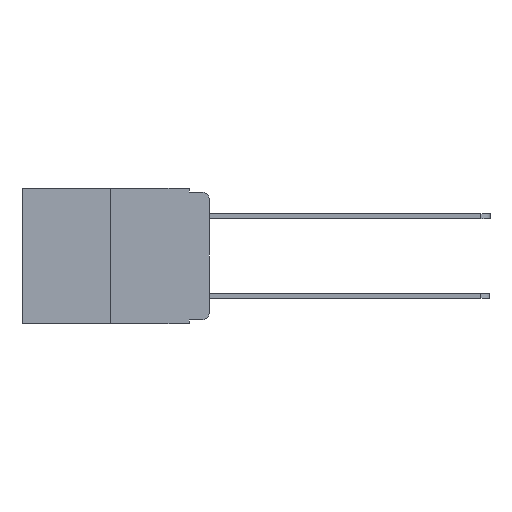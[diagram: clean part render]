
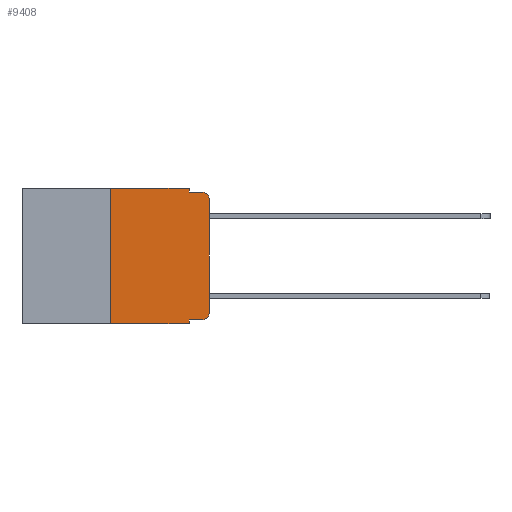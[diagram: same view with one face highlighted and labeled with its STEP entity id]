
A CAD part, left-side view. The second image highlights one B-rep face of the part: STEP entity #9408.
In plain terms, the highlighted planar face has unit normal (-1, 0, 0).
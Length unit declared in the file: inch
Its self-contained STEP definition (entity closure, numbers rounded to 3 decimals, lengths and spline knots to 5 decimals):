
#46 = DIRECTION ( 'NONE',  ( 0., -1., 0. ) ) ;
#135 = EDGE_CURVE ( 'NONE', #862, #12136, #13239, .T. ) ;
#237 = CARTESIAN_POINT ( 'NONE',  ( 0., 0.051, -0.333 ) ) ;
#331 = CIRCLE ( 'NONE', #6655, 0.02 ) ;
#479 = LINE ( 'NONE', #8458, #13839 ) ;
#651 = VERTEX_POINT ( 'NONE', #237 ) ;
#794 = VECTOR ( 'NONE', #2720, 39.37008 ) ;
#862 = VERTEX_POINT ( 'NONE', #13949 ) ;
#1198 = CARTESIAN_POINT ( 'NONE',  ( 0., 0., -0.03 ) ) ;
#1279 = CARTESIAN_POINT ( 'NONE',  ( 0., 0., -0.313 ) ) ;
#1744 = CARTESIAN_POINT ( 'NONE',  ( 0., 0., 0. ) ) ;
#1793 = CARTESIAN_POINT ( 'NONE',  ( 0., 0.051, -0.01 ) ) ;
#2122 = DIRECTION ( 'NONE',  ( 0., 0., -1. ) ) ;
#2189 = DIRECTION ( 'NONE',  ( 0., 0., -1. ) ) ;
#2307 = EDGE_CURVE ( 'NONE', #651, #6508, #14118, .T. ) ;
#2720 = DIRECTION ( 'NONE',  ( 0., 0., -1. ) ) ;
#2886 = EDGE_CURVE ( 'NONE', #14373, #12136, #7454, .T. ) ;
#3459 = CARTESIAN_POINT ( 'NONE',  ( 0., 0.02, -0.313 ) ) ;
#3472 = EDGE_LOOP ( 'NONE', ( #11298, #11519, #11574, #11681, #11827, #10080, #9507, #10135, #4660, #4929 ) ) ;
#3650 = VECTOR ( 'NONE', #16010, 39.37008 ) ;
#3783 = EDGE_CURVE ( 'NONE', #9154, #14373, #8164, .T. ) ;
#4089 = VERTEX_POINT ( 'NONE', #15399 ) ;
#4340 = CARTESIAN_POINT ( 'NONE',  ( 0., 0.051, -0.333 ) ) ;
#4660 = ORIENTED_EDGE ( 'NONE', *, *, #9292, .T. ) ;
#4740 = DIRECTION ( 'NONE',  ( 0., 0., -1. ) ) ;
#4780 = CARTESIAN_POINT ( 'NONE',  ( 0., 0.051, 0. ) ) ;
#4929 = ORIENTED_EDGE ( 'NONE', *, *, #5244, .T. ) ;
#4959 = VECTOR ( 'NONE', #7750, 39.37008 ) ;
#5244 = EDGE_CURVE ( 'NONE', #4089, #9154, #331, .T. ) ;
#5691 = CARTESIAN_POINT ( 'NONE',  ( 0., 0.02, -0.01 ) ) ;
#6508 = VERTEX_POINT ( 'NONE', #15733 ) ;
#6655 = AXIS2_PLACEMENT_3D ( 'NONE', #3459, #12138, #4740 ) ;
#6708 = AXIS2_PLACEMENT_3D ( 'NONE', #14451, #9598, #2122 ) ;
#6870 = CARTESIAN_POINT ( 'NONE',  ( 0., 0.051, 0. ) ) ;
#7086 = VECTOR ( 'NONE', #46, 39.37008 ) ;
#7454 = CIRCLE ( 'NONE', #15289, 0.02 ) ;
#7464 = VERTEX_POINT ( 'NONE', #9015 ) ;
#7537 = VECTOR ( 'NONE', #14561, 39.37008 ) ;
#7656 = DIRECTION ( 'NONE',  ( 0., -1., 0. ) ) ;
#7750 = DIRECTION ( 'NONE',  ( 0., 0., 1. ) ) ;
#7980 = EDGE_CURVE ( 'NONE', #12337, #12923, #13455, .T. ) ;
#8140 = VECTOR ( 'NONE', #11762, 39.37008 ) ;
#8164 = LINE ( 'NONE', #1744, #4959 ) ;
#8371 = PLANE ( 'NONE',  #6708 ) ;
#8458 = CARTESIAN_POINT ( 'NONE',  ( 0., 0.25, 0. ) ) ;
#9015 = CARTESIAN_POINT ( 'NONE',  ( 0., 0.25, -0.343 ) ) ;
#9154 = VERTEX_POINT ( 'NONE', #1279 ) ;
#9292 = EDGE_CURVE ( 'NONE', #651, #4089, #15051, .T. ) ;
#9408 = ADVANCED_FACE ( 'NONE', ( #12827 ), #8371, .F. ) ;
#9507 = ORIENTED_EDGE ( 'NONE', *, *, #10607, .T. ) ;
#9598 = DIRECTION ( 'NONE',  ( 1., 0., 0. ) ) ;
#9620 = VECTOR ( 'NONE', #7656, 39.37008 ) ;
#10080 = ORIENTED_EDGE ( 'NONE', *, *, #12384, .F. ) ;
#10135 = ORIENTED_EDGE ( 'NONE', *, *, #2307, .F. ) ;
#10607 = EDGE_CURVE ( 'NONE', #7464, #6508, #14059, .T. ) ;
#10865 = LINE ( 'NONE', #4780, #7537 ) ;
#11298 = ORIENTED_EDGE ( 'NONE', *, *, #3783, .T. ) ;
#11519 = ORIENTED_EDGE ( 'NONE', *, *, #2886, .T. ) ;
#11574 = ORIENTED_EDGE ( 'NONE', *, *, #135, .F. ) ;
#11681 = ORIENTED_EDGE ( 'NONE', *, *, #15567, .F. ) ;
#11762 = DIRECTION ( 'NONE',  ( 0., -1., 0. ) ) ;
#11827 = ORIENTED_EDGE ( 'NONE', *, *, #7980, .F. ) ;
#12104 = CARTESIAN_POINT ( 'NONE',  ( 0., 0.25, 0. ) ) ;
#12136 = VERTEX_POINT ( 'NONE', #5691 ) ;
#12138 = DIRECTION ( 'NONE',  ( -1., 0., 0. ) ) ;
#12337 = VERTEX_POINT ( 'NONE', #12104 ) ;
#12384 = EDGE_CURVE ( 'NONE', #7464, #12337, #479, .T. ) ;
#12827 = FACE_OUTER_BOUND ( 'NONE', #3472, .T. ) ;
#12923 = VERTEX_POINT ( 'NONE', #14259 ) ;
#13239 = LINE ( 'NONE', #1793, #7086 ) ;
#13278 = CARTESIAN_POINT ( 'NONE',  ( 0., 0.02, -0.03 ) ) ;
#13455 = LINE ( 'NONE', #14865, #3650 ) ;
#13796 = CARTESIAN_POINT ( 'NONE',  ( 0., 0.473, -0.343 ) ) ;
#13839 = VECTOR ( 'NONE', #14580, 39.37008 ) ;
#13949 = CARTESIAN_POINT ( 'NONE',  ( 0., 0.051, -0.01 ) ) ;
#14059 = LINE ( 'NONE', #13796, #9620 ) ;
#14118 = LINE ( 'NONE', #6870, #794 ) ;
#14259 = CARTESIAN_POINT ( 'NONE',  ( 0., 0.051, 0. ) ) ;
#14373 = VERTEX_POINT ( 'NONE', #1198 ) ;
#14451 = CARTESIAN_POINT ( 'NONE',  ( 0., 0.473, 0. ) ) ;
#14561 = DIRECTION ( 'NONE',  ( 0., 0., -1. ) ) ;
#14580 = DIRECTION ( 'NONE',  ( 0., 0., 1. ) ) ;
#14865 = CARTESIAN_POINT ( 'NONE',  ( 0., 0.473, 0. ) ) ;
#15051 = LINE ( 'NONE', #4340, #8140 ) ;
#15289 = AXIS2_PLACEMENT_3D ( 'NONE', #13278, #15937, #2189 ) ;
#15399 = CARTESIAN_POINT ( 'NONE',  ( 0., 0.02, -0.333 ) ) ;
#15567 = EDGE_CURVE ( 'NONE', #12923, #862, #10865, .T. ) ;
#15733 = CARTESIAN_POINT ( 'NONE',  ( 0., 0.051, -0.343 ) ) ;
#15937 = DIRECTION ( 'NONE',  ( -1., 0., 0. ) ) ;
#16010 = DIRECTION ( 'NONE',  ( 0., -1., 0. ) ) ;
